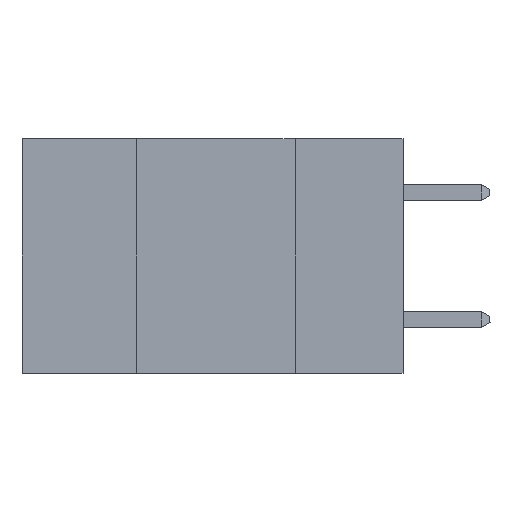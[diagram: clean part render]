
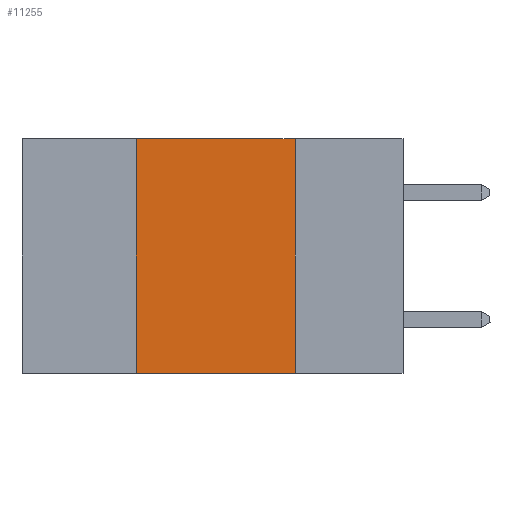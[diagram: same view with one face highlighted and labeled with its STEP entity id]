
A CAD part, left-side view. The second image highlights one B-rep face of the part: STEP entity #11255.
In plain terms, the highlighted planar face has unit normal (-1, 0, 0).
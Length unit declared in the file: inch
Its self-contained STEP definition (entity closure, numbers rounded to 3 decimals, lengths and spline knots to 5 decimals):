
#471 = DIRECTION ( 'NONE',  ( 0., -1., 0. ) ) ;
#802 = EDGE_CURVE ( 'NONE', #9275, #4707, #18721, .T. ) ;
#843 = DIRECTION ( 'NONE',  ( 0., 0., 1. ) ) ;
#1279 = EDGE_LOOP ( 'NONE', ( #23433, #19547, #7274, #18252 ) ) ;
#2335 = VERTEX_POINT ( 'NONE', #8746 ) ;
#3209 = VECTOR ( 'NONE', #843, 39.37008 ) ;
#3931 = LINE ( 'NONE', #7029, #3209 ) ;
#4490 = EDGE_CURVE ( 'NONE', #9043, #9275, #3931, .T. ) ;
#4707 = VERTEX_POINT ( 'NONE', #12645 ) ;
#5751 = DIRECTION ( 'NONE',  ( 0., -1., 0. ) ) ;
#6759 = CARTESIAN_POINT ( 'NONE',  ( 0., 0.6, -0.37 ) ) ;
#7029 = CARTESIAN_POINT ( 'NONE',  ( 0., 0.42, 0. ) ) ;
#7274 = ORIENTED_EDGE ( 'NONE', *, *, #4490, .F. ) ;
#7515 = LINE ( 'NONE', #10379, #10760 ) ;
#8746 = CARTESIAN_POINT ( 'NONE',  ( 0., 0.17, -0.37 ) ) ;
#9043 = VERTEX_POINT ( 'NONE', #9855 ) ;
#9275 = VERTEX_POINT ( 'NONE', #13875 ) ;
#9733 = DIRECTION ( 'NONE',  ( 1., 0., 0. ) ) ;
#9855 = CARTESIAN_POINT ( 'NONE',  ( 0., 0.42, -0.37 ) ) ;
#9984 = EDGE_CURVE ( 'NONE', #4707, #2335, #7515, .T. ) ;
#10142 = VECTOR ( 'NONE', #5751, 39.37008 ) ;
#10379 = CARTESIAN_POINT ( 'NONE',  ( 0., 0.17, 0. ) ) ;
#10760 = VECTOR ( 'NONE', #16390, 39.37008 ) ;
#11255 = ADVANCED_FACE ( 'NONE', ( #14276 ), #24603, .F. ) ;
#11915 = DIRECTION ( 'NONE',  ( 0., 0., -1. ) ) ;
#12645 = CARTESIAN_POINT ( 'NONE',  ( 0., 0.17, 0. ) ) ;
#13478 = VECTOR ( 'NONE', #471, 39.37008 ) ;
#13875 = CARTESIAN_POINT ( 'NONE',  ( 0., 0.42, 0. ) ) ;
#14276 = FACE_OUTER_BOUND ( 'NONE', #1279, .T. ) ;
#16390 = DIRECTION ( 'NONE',  ( 0., 0., -1. ) ) ;
#18105 = EDGE_CURVE ( 'NONE', #9043, #2335, #26694, .T. ) ;
#18252 = ORIENTED_EDGE ( 'NONE', *, *, #18105, .T. ) ;
#18721 = LINE ( 'NONE', #20552, #10142 ) ;
#19547 = ORIENTED_EDGE ( 'NONE', *, *, #802, .F. ) ;
#20552 = CARTESIAN_POINT ( 'NONE',  ( 0., 0.6, 0. ) ) ;
#22553 = AXIS2_PLACEMENT_3D ( 'NONE', #26955, #9733, #11915 ) ;
#23433 = ORIENTED_EDGE ( 'NONE', *, *, #9984, .F. ) ;
#24603 = PLANE ( 'NONE',  #22553 ) ;
#26694 = LINE ( 'NONE', #6759, #13478 ) ;
#26955 = CARTESIAN_POINT ( 'NONE',  ( 0., 0.6, 0. ) ) ;
